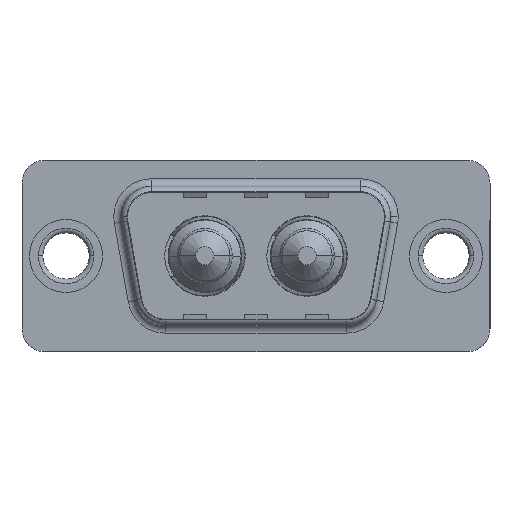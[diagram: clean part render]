
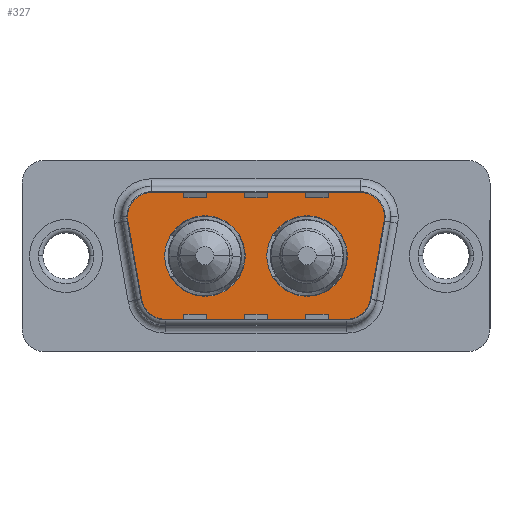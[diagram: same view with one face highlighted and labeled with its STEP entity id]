
A CAD part, top view. The second image highlights one B-rep face of the part: STEP entity #327.
In plain terms, the highlighted planar face has unit normal (0, 0, 1).
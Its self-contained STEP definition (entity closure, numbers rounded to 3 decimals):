
#4 = AXIS2_PLACEMENT_3D ( 'NONE', #2556, #7891, #9879 ) ;
#122 = ORIENTED_EDGE ( 'NONE', *, *, #2443, .T. ) ;
#148 = DIRECTION ( 'NONE',  ( -1., 0., 0. ) ) ;
#209 = AXIS2_PLACEMENT_3D ( 'NONE', #9122, #448, #3770 ) ;
#216 = ORIENTED_EDGE ( 'NONE', *, *, #6786, .F. ) ;
#227 = VERTEX_POINT ( 'NONE', #3729 ) ;
#238 = EDGE_CURVE ( 'NONE', #5271, #2881, #8712, .T. ) ;
#317 = CARTESIAN_POINT ( 'NONE',  ( 15.86, 0., 0. ) ) ;
#327 = ADVANCED_FACE ( 'NONE', ( #9526, #3449, #9289 ), #7587, .T. ) ;
#401 = DIRECTION ( 'NONE',  ( 0.174, 0.985, 0. ) ) ;
#448 = DIRECTION ( 'NONE',  ( 0., 0., 1. ) ) ;
#476 = VECTOR ( 'NONE', #401, 1000. ) ;
#497 = ORIENTED_EDGE ( 'NONE', *, *, #3427, .F. ) ;
#702 = ORIENTED_EDGE ( 'NONE', *, *, #5452, .T. ) ;
#747 = VECTOR ( 'NONE', #148, 1000. ) ;
#768 = EDGE_LOOP ( 'NONE', ( #3145, #497 ) ) ;
#968 = EDGE_CURVE ( 'NONE', #3777, #2613, #7008, .T. ) ;
#1011 = CARTESIAN_POINT ( 'NONE',  ( 3.466, 2.553, 0. ) ) ;
#1157 = CARTESIAN_POINT ( 'NONE',  ( 9.14, 0., 0. ) ) ;
#1230 = CARTESIAN_POINT ( 'NONE',  ( 21.534, 2.553, 0. ) ) ;
#1239 = AXIS2_PLACEMENT_3D ( 'NONE', #1157, #1425, #8260 ) ;
#1285 = EDGE_CURVE ( 'NONE', #8871, #9430, #5521, .T. ) ;
#1308 = EDGE_CURVE ( 'NONE', #8521, #4427, #3523, .T. ) ;
#1425 = DIRECTION ( 'NONE',  ( 0., 0., 1. ) ) ;
#1523 = CARTESIAN_POINT ( 'NONE',  ( 13.21, 0., 0. ) ) ;
#1597 = CARTESIAN_POINT ( 'NONE',  ( 21.564, 2.9, 0. ) ) ;
#1615 = CARTESIAN_POINT ( 'NONE',  ( 6.459, -2.9, 0. ) ) ;
#1757 = VECTOR ( 'NONE', #2217, 1000. ) ;
#1763 = DIRECTION ( 'NONE',  ( 0.174, -0.985, 0. ) ) ;
#2001 = LINE ( 'NONE', #3986, #1757 ) ;
#2091 = AXIS2_PLACEMENT_3D ( 'NONE', #317, #8053, #7908 ) ;
#2188 = AXIS2_PLACEMENT_3D ( 'NONE', #8732, #8214, #5919 ) ;
#2204 = CARTESIAN_POINT ( 'NONE',  ( 19.564, 2.9, 0. ) ) ;
#2217 = DIRECTION ( 'NONE',  ( 1., 0., 0. ) ) ;
#2443 = EDGE_CURVE ( 'NONE', #2613, #8259, #3015, .T. ) ;
#2556 = CARTESIAN_POINT ( 'NONE',  ( 18.541, -2.9, 0. ) ) ;
#2613 = VERTEX_POINT ( 'NONE', #6627 ) ;
#2827 = CIRCLE ( 'NONE', #7969, 2.65 ) ;
#2841 = AXIS2_PLACEMENT_3D ( 'NONE', #9262, #8298, #5744 ) ;
#2881 = VERTEX_POINT ( 'NONE', #1523 ) ;
#2939 = CIRCLE ( 'NONE', #5375, 2. ) ;
#3009 = ORIENTED_EDGE ( 'NONE', *, *, #9886, .T. ) ;
#3015 = LINE ( 'NONE', #6353, #747 ) ;
#3145 = ORIENTED_EDGE ( 'NONE', *, *, #1285, .F. ) ;
#3260 = VERTEX_POINT ( 'NONE', #9719 ) ;
#3321 = EDGE_CURVE ( 'NONE', #8259, #3260, #9638, .T. ) ;
#3405 = DIRECTION ( 'NONE',  ( -1., 0., 0. ) ) ;
#3426 = ORIENTED_EDGE ( 'NONE', *, *, #7916, .T. ) ;
#3427 = EDGE_CURVE ( 'NONE', #9430, #8871, #2827, .T. ) ;
#3449 = FACE_BOUND ( 'NONE', #768, .T. ) ;
#3523 = CIRCLE ( 'NONE', #209, 2. ) ;
#3650 = CARTESIAN_POINT ( 'NONE',  ( 18.541, -4.9, 0. ) ) ;
#3684 = EDGE_CURVE ( 'NONE', #7885, #3777, #2939, .T. ) ;
#3729 = CARTESIAN_POINT ( 'NONE',  ( 4.489, -3.247, 0. ) ) ;
#3768 = ORIENTED_EDGE ( 'NONE', *, *, #1308, .T. ) ;
#3770 = DIRECTION ( 'NONE',  ( 1., 0., 0. ) ) ;
#3777 = VERTEX_POINT ( 'NONE', #1597 ) ;
#3860 = ORIENTED_EDGE ( 'NONE', *, *, #968, .T. ) ;
#3884 = DIRECTION ( 'NONE',  ( 0., 0., 1. ) ) ;
#3986 = CARTESIAN_POINT ( 'NONE',  ( 6.459, -4.9, 0. ) ) ;
#4188 = CARTESIAN_POINT ( 'NONE',  ( 11.79, 0., 0. ) ) ;
#4395 = ORIENTED_EDGE ( 'NONE', *, *, #3321, .T. ) ;
#4427 = VERTEX_POINT ( 'NONE', #8896 ) ;
#4520 = LINE ( 'NONE', #1011, #8365 ) ;
#4783 = CARTESIAN_POINT ( 'NONE',  ( 6.459, -4.9, 0. ) ) ;
#4818 = DIRECTION ( 'NONE',  ( 1., 0., 0. ) ) ;
#4906 = ORIENTED_EDGE ( 'NONE', *, *, #3684, .T. ) ;
#5039 = DIRECTION ( 'NONE',  ( 0., 0., 1. ) ) ;
#5271 = VERTEX_POINT ( 'NONE', #9242 ) ;
#5375 = AXIS2_PLACEMENT_3D ( 'NONE', #2204, #3884, #8468 ) ;
#5383 = CARTESIAN_POINT ( 'NONE',  ( 21.534, 2.553, 0. ) ) ;
#5452 = EDGE_CURVE ( 'NONE', #4427, #7885, #6566, .T. ) ;
#5521 = CIRCLE ( 'NONE', #1239, 2.65 ) ;
#5721 = VERTEX_POINT ( 'NONE', #4783 ) ;
#5744 = DIRECTION ( 'NONE',  ( 1., 0., 0. ) ) ;
#5919 = DIRECTION ( 'NONE',  ( -1., 0., 0. ) ) ;
#6063 = CARTESIAN_POINT ( 'NONE',  ( 9.14, 0., 0. ) ) ;
#6082 = CARTESIAN_POINT ( 'NONE',  ( 5.436, 4.9, 0. ) ) ;
#6353 = CARTESIAN_POINT ( 'NONE',  ( 5.436, 4.9, 0. ) ) ;
#6566 = LINE ( 'NONE', #1230, #476 ) ;
#6627 = CARTESIAN_POINT ( 'NONE',  ( 19.564, 4.9, 0. ) ) ;
#6679 = DIRECTION ( 'NONE',  ( 0., 0., 1. ) ) ;
#6786 = EDGE_CURVE ( 'NONE', #2881, #5271, #9644, .T. ) ;
#7008 = CIRCLE ( 'NONE', #2188, 2. ) ;
#7228 = AXIS2_PLACEMENT_3D ( 'NONE', #7830, #5039, #8265 ) ;
#7291 = EDGE_CURVE ( 'NONE', #5721, #8521, #2001, .T. ) ;
#7466 = AXIS2_PLACEMENT_3D ( 'NONE', #1615, #7965, #3405 ) ;
#7587 = PLANE ( 'NONE',  #4 ) ;
#7830 = CARTESIAN_POINT ( 'NONE',  ( 15.86, 0., 0. ) ) ;
#7885 = VERTEX_POINT ( 'NONE', #5383 ) ;
#7891 = DIRECTION ( 'NONE',  ( 0., 0., 1. ) ) ;
#7908 = DIRECTION ( 'NONE',  ( 1., 0., 0. ) ) ;
#7916 = EDGE_CURVE ( 'NONE', #227, #5721, #9288, .T. ) ;
#7965 = DIRECTION ( 'NONE',  ( 0., 0., 1. ) ) ;
#7969 = AXIS2_PLACEMENT_3D ( 'NONE', #6063, #6679, #4818 ) ;
#8053 = DIRECTION ( 'NONE',  ( 0., 0., 1. ) ) ;
#8121 = EDGE_LOOP ( 'NONE', ( #3768, #702, #4906, #3860, #122, #4395, #3009, #3426, #9450 ) ) ;
#8214 = DIRECTION ( 'NONE',  ( 0., 0., 1. ) ) ;
#8259 = VERTEX_POINT ( 'NONE', #6082 ) ;
#8260 = DIRECTION ( 'NONE',  ( 1., 0., 0. ) ) ;
#8265 = DIRECTION ( 'NONE',  ( 1., 0., 0. ) ) ;
#8298 = DIRECTION ( 'NONE',  ( 0., 0., 1. ) ) ;
#8365 = VECTOR ( 'NONE', #1763, 1000. ) ;
#8468 = DIRECTION ( 'NONE',  ( -1., 0., 0. ) ) ;
#8521 = VERTEX_POINT ( 'NONE', #3650 ) ;
#8712 = CIRCLE ( 'NONE', #7228, 2.65 ) ;
#8732 = CARTESIAN_POINT ( 'NONE',  ( 19.564, 2.9, 0. ) ) ;
#8871 = VERTEX_POINT ( 'NONE', #4188 ) ;
#8896 = CARTESIAN_POINT ( 'NONE',  ( 20.511, -3.247, 0. ) ) ;
#9029 = ORIENTED_EDGE ( 'NONE', *, *, #238, .F. ) ;
#9122 = CARTESIAN_POINT ( 'NONE',  ( 18.541, -2.9, 0. ) ) ;
#9242 = CARTESIAN_POINT ( 'NONE',  ( 18.51, 0., 0. ) ) ;
#9262 = CARTESIAN_POINT ( 'NONE',  ( 5.436, 2.9, 0. ) ) ;
#9288 = CIRCLE ( 'NONE', #7466, 2. ) ;
#9289 = FACE_OUTER_BOUND ( 'NONE', #8121, .T. ) ;
#9430 = VERTEX_POINT ( 'NONE', #9511 ) ;
#9450 = ORIENTED_EDGE ( 'NONE', *, *, #7291, .T. ) ;
#9511 = CARTESIAN_POINT ( 'NONE',  ( 6.49, 0., 0. ) ) ;
#9526 = FACE_BOUND ( 'NONE', #9844, .T. ) ;
#9638 = CIRCLE ( 'NONE', #2841, 2. ) ;
#9644 = CIRCLE ( 'NONE', #2091, 2.65 ) ;
#9719 = CARTESIAN_POINT ( 'NONE',  ( 3.466, 2.553, 0. ) ) ;
#9844 = EDGE_LOOP ( 'NONE', ( #9029, #216 ) ) ;
#9879 = DIRECTION ( 'NONE',  ( 1., 0., 0. ) ) ;
#9886 = EDGE_CURVE ( 'NONE', #3260, #227, #4520, .T. ) ;
